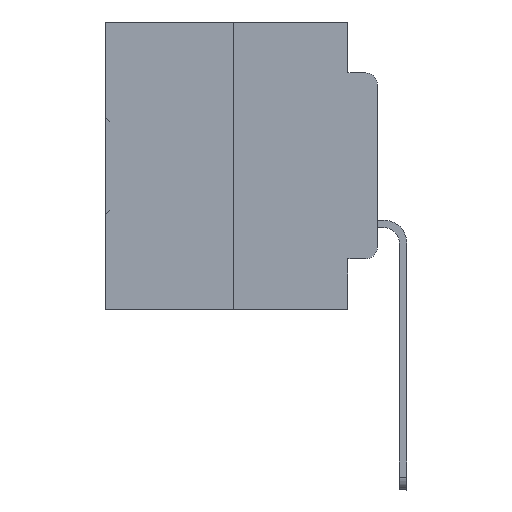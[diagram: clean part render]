
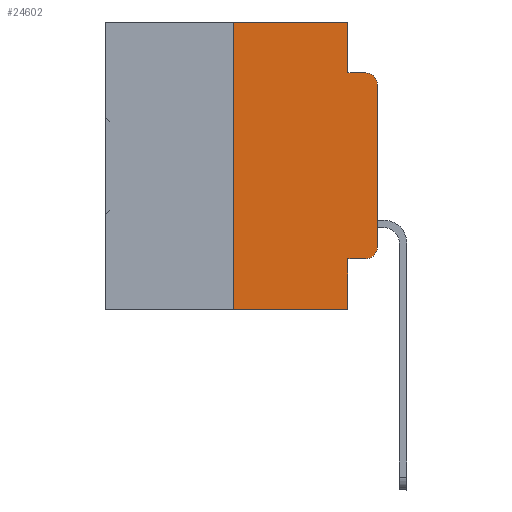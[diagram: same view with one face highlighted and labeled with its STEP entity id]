
A CAD part, left-side view. The second image highlights one B-rep face of the part: STEP entity #24602.
In plain terms, the highlighted planar face has unit normal (-1, 0, 0).
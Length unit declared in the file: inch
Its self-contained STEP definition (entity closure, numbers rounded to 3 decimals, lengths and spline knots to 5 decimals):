
#392 = DIRECTION ( 'NONE',  ( 0., -1., 0. ) ) ;
#1030 = LINE ( 'NONE', #6122, #14449 ) ;
#1305 = CARTESIAN_POINT ( 'NONE',  ( 0., 0.051, 0. ) ) ;
#1351 = CARTESIAN_POINT ( 'NONE',  ( 0., 0.02, -0.0885 ) ) ;
#1906 = VERTEX_POINT ( 'NONE', #29613 ) ;
#2345 = EDGE_CURVE ( 'NONE', #27561, #1906, #34023, .T. ) ;
#2372 = DIRECTION ( 'NONE',  ( 0., 0., -1. ) ) ;
#2616 = VECTOR ( 'NONE', #12003, 39.37008 ) ;
#3085 = CIRCLE ( 'NONE', #12617, 0.02 ) ;
#3300 = DIRECTION ( 'NONE',  ( 1., 0., 0. ) ) ;
#3309 = CARTESIAN_POINT ( 'NONE',  ( 0., 0.051, -0.5 ) ) ;
#3329 = AXIS2_PLACEMENT_3D ( 'NONE', #25241, #3300, #32778 ) ;
#3335 = CARTESIAN_POINT ( 'NONE',  ( 0., 0.051, -0.0885 ) ) ;
#3531 = CARTESIAN_POINT ( 'NONE',  ( 0., 0.051, -0.4115 ) ) ;
#3682 = EDGE_CURVE ( 'NONE', #22965, #12375, #20981, .T. ) ;
#3878 = DIRECTION ( 'NONE',  ( 0., 0., 1. ) ) ;
#5022 = DIRECTION ( 'NONE',  ( 0., -1., 0. ) ) ;
#5059 = CARTESIAN_POINT ( 'NONE',  ( 0., 0.051, 0. ) ) ;
#6122 = CARTESIAN_POINT ( 'NONE',  ( 0., 0.051, -0.0885 ) ) ;
#6415 = CARTESIAN_POINT ( 'NONE',  ( 0., 0.02, -0.1085 ) ) ;
#6571 = EDGE_CURVE ( 'NONE', #19440, #13925, #21175, .T. ) ;
#6847 = ORIENTED_EDGE ( 'NONE', *, *, #29037, .T. ) ;
#7216 = LINE ( 'NONE', #12136, #28087 ) ;
#7577 = CARTESIAN_POINT ( 'NONE',  ( 0., 0.25, -0.5 ) ) ;
#7980 = VERTEX_POINT ( 'NONE', #30474 ) ;
#8549 = EDGE_CURVE ( 'NONE', #13925, #22990, #9713, .T. ) ;
#9713 = LINE ( 'NONE', #1305, #2616 ) ;
#10267 = ORIENTED_EDGE ( 'NONE', *, *, #8549, .F. ) ;
#11171 = EDGE_CURVE ( 'NONE', #22990, #16355, #1030, .T. ) ;
#11620 = AXIS2_PLACEMENT_3D ( 'NONE', #13893, #32148, #24605 ) ;
#11687 = DIRECTION ( 'NONE',  ( -1., 0., 0. ) ) ;
#12003 = DIRECTION ( 'NONE',  ( 0., 0., -1. ) ) ;
#12136 = CARTESIAN_POINT ( 'NONE',  ( 0., 0., 0. ) ) ;
#12375 = VERTEX_POINT ( 'NONE', #3309 ) ;
#12617 = AXIS2_PLACEMENT_3D ( 'NONE', #6415, #11687, #14311 ) ;
#13893 = CARTESIAN_POINT ( 'NONE',  ( 0., 0.02, -0.3915 ) ) ;
#13925 = VERTEX_POINT ( 'NONE', #5059 ) ;
#14311 = DIRECTION ( 'NONE',  ( 0., 0., -1. ) ) ;
#14449 = VECTOR ( 'NONE', #19812, 39.37008 ) ;
#14630 = LINE ( 'NONE', #23391, #31001 ) ;
#15795 = VECTOR ( 'NONE', #392, 39.37008 ) ;
#16355 = VERTEX_POINT ( 'NONE', #1351 ) ;
#16672 = PLANE ( 'NONE',  #3329 ) ;
#17195 = LINE ( 'NONE', #33303, #23533 ) ;
#17634 = VECTOR ( 'NONE', #5022, 39.37008 ) ;
#18072 = ORIENTED_EDGE ( 'NONE', *, *, #3682, .F. ) ;
#18250 = ORIENTED_EDGE ( 'NONE', *, *, #2345, .T. ) ;
#19239 = VERTEX_POINT ( 'NONE', #7577 ) ;
#19440 = VERTEX_POINT ( 'NONE', #30885 ) ;
#19812 = DIRECTION ( 'NONE',  ( 0., -1., 0. ) ) ;
#20305 = EDGE_CURVE ( 'NONE', #7980, #16355, #3085, .T. ) ;
#20414 = DIRECTION ( 'NONE',  ( 0., 0., 1. ) ) ;
#20981 = LINE ( 'NONE', #34295, #32145 ) ;
#21175 = LINE ( 'NONE', #31691, #17634 ) ;
#22965 = VERTEX_POINT ( 'NONE', #32993 ) ;
#22990 = VERTEX_POINT ( 'NONE', #3335 ) ;
#23391 = CARTESIAN_POINT ( 'NONE',  ( 0., 0.25, 0. ) ) ;
#23533 = VECTOR ( 'NONE', #33143, 39.37008 ) ;
#24602 = ADVANCED_FACE ( 'NONE', ( #27339 ), #16672, .F. ) ;
#24605 = DIRECTION ( 'NONE',  ( 0., 0., -1. ) ) ;
#25241 = CARTESIAN_POINT ( 'NONE',  ( 0., 0.473, 0. ) ) ;
#26539 = EDGE_LOOP ( 'NONE', ( #34510, #29211, #32567, #10267, #26687, #31747, #6847, #18072, #29812, #18250 ) ) ;
#26687 = ORIENTED_EDGE ( 'NONE', *, *, #6571, .F. ) ;
#27339 = FACE_OUTER_BOUND ( 'NONE', #26539, .T. ) ;
#27561 = VERTEX_POINT ( 'NONE', #29127 ) ;
#27582 = LINE ( 'NONE', #3531, #15795 ) ;
#28087 = VECTOR ( 'NONE', #3878, 39.37008 ) ;
#28800 = EDGE_CURVE ( 'NONE', #19239, #19440, #14630, .T. ) ;
#29037 = EDGE_CURVE ( 'NONE', #19239, #12375, #17195, .T. ) ;
#29127 = CARTESIAN_POINT ( 'NONE',  ( 0., 0.02, -0.4115 ) ) ;
#29211 = ORIENTED_EDGE ( 'NONE', *, *, #20305, .T. ) ;
#29613 = CARTESIAN_POINT ( 'NONE',  ( 0., 0., -0.3915 ) ) ;
#29812 = ORIENTED_EDGE ( 'NONE', *, *, #30350, .T. ) ;
#30350 = EDGE_CURVE ( 'NONE', #22965, #27561, #27582, .T. ) ;
#30387 = EDGE_CURVE ( 'NONE', #1906, #7980, #7216, .T. ) ;
#30474 = CARTESIAN_POINT ( 'NONE',  ( 0., 0., -0.1085 ) ) ;
#30885 = CARTESIAN_POINT ( 'NONE',  ( 0., 0.25, 0. ) ) ;
#31001 = VECTOR ( 'NONE', #20414, 39.37008 ) ;
#31691 = CARTESIAN_POINT ( 'NONE',  ( 0., 0.473, 0. ) ) ;
#31747 = ORIENTED_EDGE ( 'NONE', *, *, #28800, .F. ) ;
#32145 = VECTOR ( 'NONE', #2372, 39.37008 ) ;
#32148 = DIRECTION ( 'NONE',  ( -1., 0., 0. ) ) ;
#32567 = ORIENTED_EDGE ( 'NONE', *, *, #11171, .F. ) ;
#32778 = DIRECTION ( 'NONE',  ( 0., 0., -1. ) ) ;
#32993 = CARTESIAN_POINT ( 'NONE',  ( 0., 0.051, -0.4115 ) ) ;
#33143 = DIRECTION ( 'NONE',  ( 0., -1., 0. ) ) ;
#33303 = CARTESIAN_POINT ( 'NONE',  ( 0., 0.473, -0.5 ) ) ;
#34023 = CIRCLE ( 'NONE', #11620, 0.02 ) ;
#34295 = CARTESIAN_POINT ( 'NONE',  ( 0., 0.051, 0. ) ) ;
#34510 = ORIENTED_EDGE ( 'NONE', *, *, #30387, .T. ) ;
